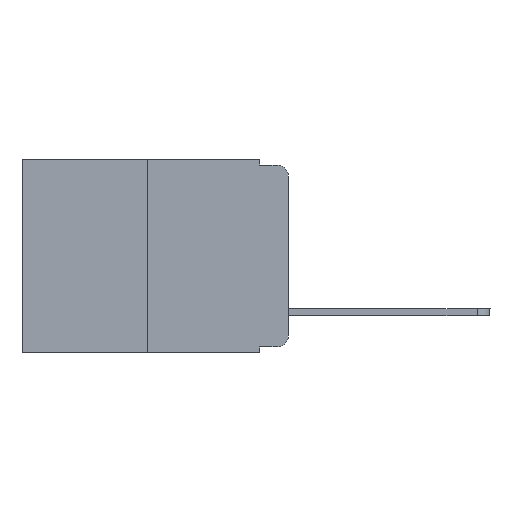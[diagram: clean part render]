
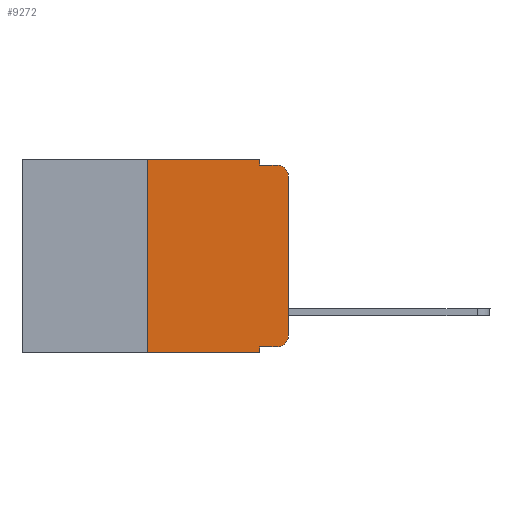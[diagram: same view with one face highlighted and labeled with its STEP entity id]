
A CAD part, left-side view. The second image highlights one B-rep face of the part: STEP entity #9272.
In plain terms, the highlighted planar face has unit normal (-1, 0, 0).
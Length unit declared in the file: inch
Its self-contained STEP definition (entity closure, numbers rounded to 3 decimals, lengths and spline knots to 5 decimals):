
#269 = DIRECTION ( 'NONE',  ( 0., 0., 1. ) ) ;
#329 = CARTESIAN_POINT ( 'NONE',  ( 0., 0., 0. ) ) ;
#461 = CARTESIAN_POINT ( 'NONE',  ( 0., 0.02, -0.333 ) ) ;
#462 = CARTESIAN_POINT ( 'NONE',  ( 0., 0.25, 0. ) ) ;
#626 = CARTESIAN_POINT ( 'NONE',  ( 0., 0., -0.03 ) ) ;
#814 = EDGE_CURVE ( 'NONE', #1369, #20486, #13596, .T. ) ;
#1258 = CARTESIAN_POINT ( 'NONE',  ( 0., 0.473, -0.343 ) ) ;
#1369 = VERTEX_POINT ( 'NONE', #16649 ) ;
#1502 = CIRCLE ( 'NONE', #14543, 0.02 ) ;
#2406 = DIRECTION ( 'NONE',  ( 0., 0., -1. ) ) ;
#2564 = VERTEX_POINT ( 'NONE', #626 ) ;
#2968 = LINE ( 'NONE', #3083, #22868 ) ;
#3083 = CARTESIAN_POINT ( 'NONE',  ( 0., 0.051, 0. ) ) ;
#4127 = CIRCLE ( 'NONE', #13104, 0.02 ) ;
#4188 = DIRECTION ( 'NONE',  ( -1., 0., 0. ) ) ;
#4642 = EDGE_CURVE ( 'NONE', #23552, #14843, #1502, .T. ) ;
#4740 = DIRECTION ( 'NONE',  ( 0., 0., -1. ) ) ;
#5006 = CARTESIAN_POINT ( 'NONE',  ( 0., 0.051, 0. ) ) ;
#5599 = DIRECTION ( 'NONE',  ( 0., -1., 0. ) ) ;
#5726 = VERTEX_POINT ( 'NONE', #6958 ) ;
#5752 = VECTOR ( 'NONE', #4740, 39.37008 ) ;
#5891 = VERTEX_POINT ( 'NONE', #21307 ) ;
#6027 = CARTESIAN_POINT ( 'NONE',  ( 0., 0.051, -0.333 ) ) ;
#6716 = ORIENTED_EDGE ( 'NONE', *, *, #12793, .T. ) ;
#6871 = CARTESIAN_POINT ( 'NONE',  ( 0., 0.02, -0.313 ) ) ;
#6958 = CARTESIAN_POINT ( 'NONE',  ( 0., 0.25, -0.343 ) ) ;
#7213 = CARTESIAN_POINT ( 'NONE',  ( 0., 0.473, 0. ) ) ;
#7386 = CARTESIAN_POINT ( 'NONE',  ( 0., 0.051, -0.343 ) ) ;
#7814 = LINE ( 'NONE', #12085, #20147 ) ;
#8216 = ORIENTED_EDGE ( 'NONE', *, *, #12317, .F. ) ;
#9041 = LINE ( 'NONE', #16686, #21330 ) ;
#9125 = VERTEX_POINT ( 'NONE', #7386 ) ;
#9272 = ADVANCED_FACE ( 'NONE', ( #16368 ), #18655, .F. ) ;
#9295 = EDGE_CURVE ( 'NONE', #16095, #5891, #17837, .T. ) ;
#9837 = AXIS2_PLACEMENT_3D ( 'NONE', #16791, #22331, #22425 ) ;
#10505 = EDGE_CURVE ( 'NONE', #14843, #2564, #21741, .T. ) ;
#10829 = ORIENTED_EDGE ( 'NONE', *, *, #9295, .F. ) ;
#10842 = EDGE_CURVE ( 'NONE', #5891, #1369, #15679, .T. ) ;
#11076 = DIRECTION ( 'NONE',  ( 0., -1., 0. ) ) ;
#12025 = CARTESIAN_POINT ( 'NONE',  ( 0., 0.02, -0.03 ) ) ;
#12085 = CARTESIAN_POINT ( 'NONE',  ( 0., 0.25, 0. ) ) ;
#12317 = EDGE_CURVE ( 'NONE', #16209, #9125, #2968, .T. ) ;
#12518 = EDGE_CURVE ( 'NONE', #5726, #16095, #7814, .T. ) ;
#12712 = ORIENTED_EDGE ( 'NONE', *, *, #10505, .T. ) ;
#12785 = EDGE_CURVE ( 'NONE', #16209, #23552, #9041, .T. ) ;
#12793 = EDGE_CURVE ( 'NONE', #5726, #9125, #17399, .T. ) ;
#12999 = EDGE_CURVE ( 'NONE', #2564, #20486, #4127, .T. ) ;
#13104 = AXIS2_PLACEMENT_3D ( 'NONE', #12025, #4188, #2406 ) ;
#13447 = ORIENTED_EDGE ( 'NONE', *, *, #814, .F. ) ;
#13596 = LINE ( 'NONE', #15403, #23229 ) ;
#13765 = VECTOR ( 'NONE', #21066, 39.37008 ) ;
#14121 = EDGE_LOOP ( 'NONE', ( #12712, #19103, #13447, #20563, #10829, #14625, #6716, #8216, #18703, #18252 ) ) ;
#14543 = AXIS2_PLACEMENT_3D ( 'NONE', #6871, #22180, #22097 ) ;
#14625 = ORIENTED_EDGE ( 'NONE', *, *, #12518, .F. ) ;
#14843 = VERTEX_POINT ( 'NONE', #24049 ) ;
#15403 = CARTESIAN_POINT ( 'NONE',  ( 0., 0.051, -0.01 ) ) ;
#15452 = VECTOR ( 'NONE', #20675, 39.37008 ) ;
#15679 = LINE ( 'NONE', #5006, #5752 ) ;
#16095 = VERTEX_POINT ( 'NONE', #462 ) ;
#16209 = VERTEX_POINT ( 'NONE', #6027 ) ;
#16368 = FACE_OUTER_BOUND ( 'NONE', #14121, .T. ) ;
#16649 = CARTESIAN_POINT ( 'NONE',  ( 0., 0.051, -0.01 ) ) ;
#16686 = CARTESIAN_POINT ( 'NONE',  ( 0., 0.051, -0.333 ) ) ;
#16791 = CARTESIAN_POINT ( 'NONE',  ( 0., 0.473, 0. ) ) ;
#16937 = CARTESIAN_POINT ( 'NONE',  ( 0., 0.02, -0.01 ) ) ;
#17399 = LINE ( 'NONE', #1258, #13765 ) ;
#17837 = LINE ( 'NONE', #7213, #15452 ) ;
#18252 = ORIENTED_EDGE ( 'NONE', *, *, #4642, .T. ) ;
#18655 = PLANE ( 'NONE',  #9837 ) ;
#18703 = ORIENTED_EDGE ( 'NONE', *, *, #12785, .T. ) ;
#19103 = ORIENTED_EDGE ( 'NONE', *, *, #12999, .T. ) ;
#20147 = VECTOR ( 'NONE', #269, 39.37008 ) ;
#20486 = VERTEX_POINT ( 'NONE', #16937 ) ;
#20563 = ORIENTED_EDGE ( 'NONE', *, *, #10842, .F. ) ;
#20675 = DIRECTION ( 'NONE',  ( 0., -1., 0. ) ) ;
#21066 = DIRECTION ( 'NONE',  ( 0., -1., 0. ) ) ;
#21166 = VECTOR ( 'NONE', #23104, 39.37008 ) ;
#21307 = CARTESIAN_POINT ( 'NONE',  ( 0., 0.051, 0. ) ) ;
#21330 = VECTOR ( 'NONE', #11076, 39.37008 ) ;
#21741 = LINE ( 'NONE', #329, #21166 ) ;
#22097 = DIRECTION ( 'NONE',  ( 0., 0., -1. ) ) ;
#22180 = DIRECTION ( 'NONE',  ( -1., 0., 0. ) ) ;
#22331 = DIRECTION ( 'NONE',  ( 1., 0., 0. ) ) ;
#22425 = DIRECTION ( 'NONE',  ( 0., 0., -1. ) ) ;
#22868 = VECTOR ( 'NONE', #24568, 39.37008 ) ;
#23104 = DIRECTION ( 'NONE',  ( 0., 0., 1. ) ) ;
#23229 = VECTOR ( 'NONE', #5599, 39.37008 ) ;
#23552 = VERTEX_POINT ( 'NONE', #461 ) ;
#24049 = CARTESIAN_POINT ( 'NONE',  ( 0., 0., -0.313 ) ) ;
#24568 = DIRECTION ( 'NONE',  ( 0., 0., -1. ) ) ;
